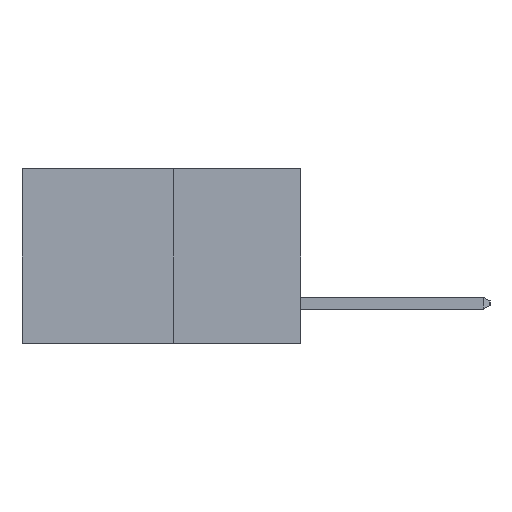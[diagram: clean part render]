
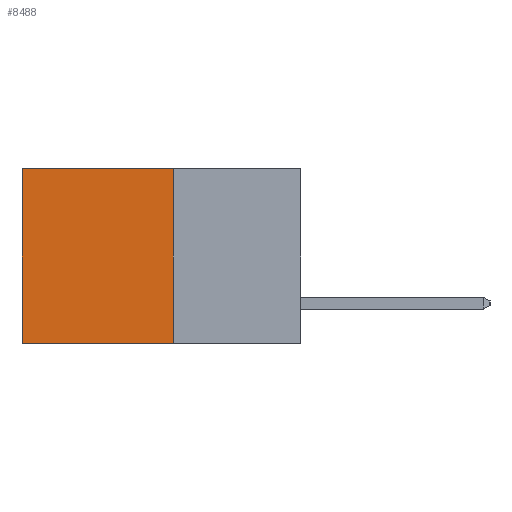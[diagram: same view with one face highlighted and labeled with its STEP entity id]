
A CAD part, left-side view. The second image highlights one B-rep face of the part: STEP entity #8488.
In plain terms, the highlighted planar face has unit normal (-1, 0, 0).
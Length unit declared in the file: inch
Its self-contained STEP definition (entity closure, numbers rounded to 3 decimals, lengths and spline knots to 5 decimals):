
#599 = DIRECTION ( 'NONE',  ( 0., 1., 0. ) ) ;
#681 = CARTESIAN_POINT ( 'NONE',  ( 0.277, 0.27, -0.37 ) ) ;
#695 = ORIENTED_EDGE ( 'NONE', *, *, #16392, .T. ) ;
#1651 = AXIS2_PLACEMENT_3D ( 'NONE', #2148, #2144, #2118 ) ;
#2118 = DIRECTION ( 'NONE',  ( 0., 0., -1. ) ) ;
#2144 = DIRECTION ( 'NONE',  ( 1., 0., 0. ) ) ;
#2148 = CARTESIAN_POINT ( 'NONE',  ( 0.277, 0.27, -0.37 ) ) ;
#2302 = PLANE ( 'NONE',  #1651 ) ;
#4053 = FACE_OUTER_BOUND ( 'NONE', #19752, .T. ) ;
#4888 = CARTESIAN_POINT ( 'NONE',  ( 0.277, 0.27, 0. ) ) ;
#5848 = ORIENTED_EDGE ( 'NONE', *, *, #14016, .F. ) ;
#6979 = CARTESIAN_POINT ( 'NONE',  ( 0.277, 0.27, -0.37 ) ) ;
#8488 = ADVANCED_FACE ( 'NONE', ( #4053 ), #2302, .F. ) ;
#9206 = DIRECTION ( 'NONE',  ( 0., 1., 0. ) ) ;
#9636 = VECTOR ( 'NONE', #599, 39.37008 ) ;
#11946 = EDGE_CURVE ( 'NONE', #23807, #22963, #20237, .T. ) ;
#14016 = EDGE_CURVE ( 'NONE', #21342, #23807, #27835, .T. ) ;
#14472 = LINE ( 'NONE', #21383, #25276 ) ;
#14932 = DIRECTION ( 'NONE',  ( 0., 0., -1. ) ) ;
#15450 = LINE ( 'NONE', #4888, #9636 ) ;
#16392 = EDGE_CURVE ( 'NONE', #24057, #22963, #14472, .T. ) ;
#18068 = CARTESIAN_POINT ( 'NONE',  ( 0.277, 0.27, 0. ) ) ;
#19752 = EDGE_LOOP ( 'NONE', ( #695, #24912, #5848, #21498 ) ) ;
#20027 = EDGE_CURVE ( 'NONE', #21342, #24057, #15450, .T. ) ;
#20237 = LINE ( 'NONE', #6979, #27962 ) ;
#21342 = VERTEX_POINT ( 'NONE', #18068 ) ;
#21383 = CARTESIAN_POINT ( 'NONE',  ( 0.277, 0.59, -0.37 ) ) ;
#21498 = ORIENTED_EDGE ( 'NONE', *, *, #20027, .T. ) ;
#22124 = CARTESIAN_POINT ( 'NONE',  ( 0.277, 0.59, 0. ) ) ;
#22489 = DIRECTION ( 'NONE',  ( 0., 0., -1. ) ) ;
#22963 = VERTEX_POINT ( 'NONE', #25827 ) ;
#23807 = VERTEX_POINT ( 'NONE', #25123 ) ;
#24057 = VERTEX_POINT ( 'NONE', #22124 ) ;
#24912 = ORIENTED_EDGE ( 'NONE', *, *, #11946, .F. ) ;
#25123 = CARTESIAN_POINT ( 'NONE',  ( 0.277, 0.27, -0.37 ) ) ;
#25276 = VECTOR ( 'NONE', #14932, 39.37008 ) ;
#25827 = CARTESIAN_POINT ( 'NONE',  ( 0.277, 0.59, -0.37 ) ) ;
#27185 = VECTOR ( 'NONE', #22489, 39.37008 ) ;
#27835 = LINE ( 'NONE', #681, #27185 ) ;
#27962 = VECTOR ( 'NONE', #9206, 39.37008 ) ;
